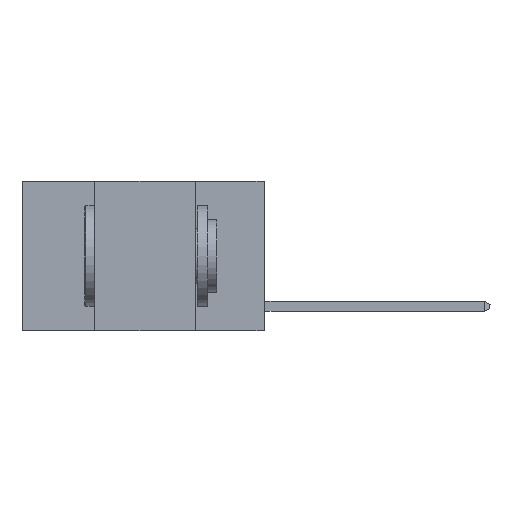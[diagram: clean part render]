
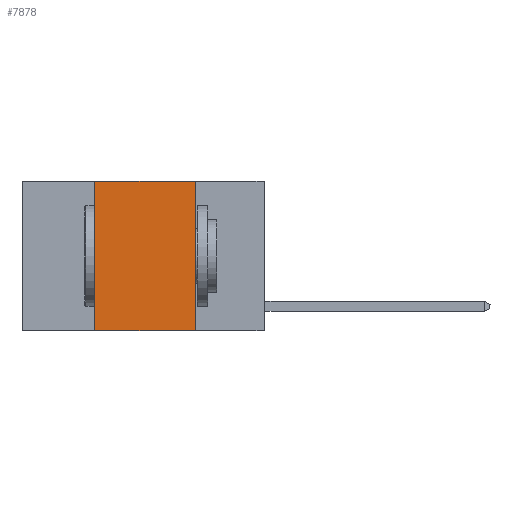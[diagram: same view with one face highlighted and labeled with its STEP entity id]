
A CAD part, left-side view. The second image highlights one B-rep face of the part: STEP entity #7878.
In plain terms, the highlighted planar face has unit normal (-1, 0, 0).
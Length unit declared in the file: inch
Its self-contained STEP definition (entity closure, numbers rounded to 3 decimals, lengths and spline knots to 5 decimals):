
#186 = CARTESIAN_POINT ( 'NONE',  ( 0., 0.42, 0. ) ) ;
#223 = ORIENTED_EDGE ( 'NONE', *, *, #13637, .T. ) ;
#840 = VERTEX_POINT ( 'NONE', #186 ) ;
#1335 = LINE ( 'NONE', #3880, #15073 ) ;
#2754 = CARTESIAN_POINT ( 'NONE',  ( 0., 0.6, -0.37 ) ) ;
#2783 = EDGE_LOOP ( 'NONE', ( #4448, #7517, #7709, #223 ) ) ;
#3258 = VECTOR ( 'NONE', #16429, 39.37008 ) ;
#3678 = VERTEX_POINT ( 'NONE', #16494 ) ;
#3880 = CARTESIAN_POINT ( 'NONE',  ( 0., 0.6, 0. ) ) ;
#4125 = LINE ( 'NONE', #15182, #3258 ) ;
#4140 = DIRECTION ( 'NONE',  ( 0., -1., 0. ) ) ;
#4448 = ORIENTED_EDGE ( 'NONE', *, *, #16670, .F. ) ;
#4880 = VECTOR ( 'NONE', #4140, 39.37008 ) ;
#6752 = VECTOR ( 'NONE', #16840, 39.37008 ) ;
#6833 = PLANE ( 'NONE',  #12660 ) ;
#7263 = CARTESIAN_POINT ( 'NONE',  ( 0., 0.17, 0. ) ) ;
#7517 = ORIENTED_EDGE ( 'NONE', *, *, #8432, .F. ) ;
#7709 = ORIENTED_EDGE ( 'NONE', *, *, #15836, .F. ) ;
#7878 = ADVANCED_FACE ( 'NONE', ( #16261 ), #6833, .F. ) ;
#8432 = EDGE_CURVE ( 'NONE', #840, #9936, #1335, .T. ) ;
#9257 = DIRECTION ( 'NONE',  ( 0., -1., 0. ) ) ;
#9517 = DIRECTION ( 'NONE',  ( 0., 0., -1. ) ) ;
#9936 = VERTEX_POINT ( 'NONE', #7263 ) ;
#10300 = VERTEX_POINT ( 'NONE', #15795 ) ;
#10424 = LINE ( 'NONE', #13046, #6752 ) ;
#11309 = DIRECTION ( 'NONE',  ( 1., 0., 0. ) ) ;
#11982 = LINE ( 'NONE', #2754, #4880 ) ;
#12660 = AXIS2_PLACEMENT_3D ( 'NONE', #15918, #11309, #9517 ) ;
#13046 = CARTESIAN_POINT ( 'NONE',  ( 0., 0.17, 0. ) ) ;
#13637 = EDGE_CURVE ( 'NONE', #3678, #10300, #11982, .T. ) ;
#15073 = VECTOR ( 'NONE', #9257, 39.37008 ) ;
#15182 = CARTESIAN_POINT ( 'NONE',  ( 0., 0.42, 0. ) ) ;
#15795 = CARTESIAN_POINT ( 'NONE',  ( 0., 0.17, -0.37 ) ) ;
#15836 = EDGE_CURVE ( 'NONE', #3678, #840, #4125, .T. ) ;
#15918 = CARTESIAN_POINT ( 'NONE',  ( 0., 0.6, 0. ) ) ;
#16261 = FACE_OUTER_BOUND ( 'NONE', #2783, .T. ) ;
#16429 = DIRECTION ( 'NONE',  ( 0., 0., 1. ) ) ;
#16494 = CARTESIAN_POINT ( 'NONE',  ( 0., 0.42, -0.37 ) ) ;
#16670 = EDGE_CURVE ( 'NONE', #9936, #10300, #10424, .T. ) ;
#16840 = DIRECTION ( 'NONE',  ( 0., 0., -1. ) ) ;
